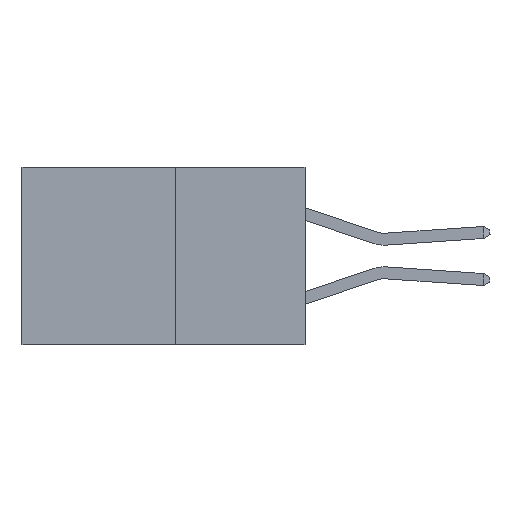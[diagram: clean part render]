
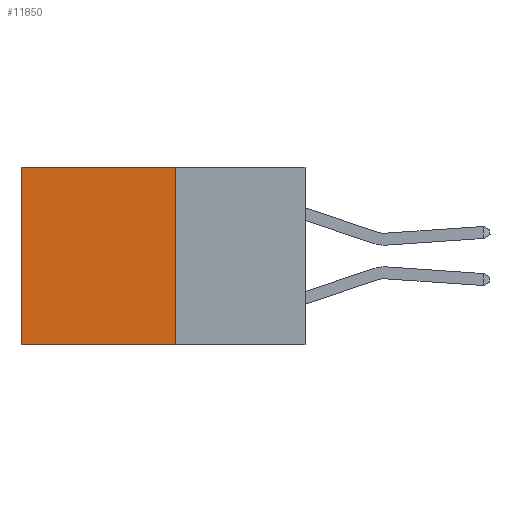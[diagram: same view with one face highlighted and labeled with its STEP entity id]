
A CAD part, left-side view. The second image highlights one B-rep face of the part: STEP entity #11850.
In plain terms, the highlighted planar face has unit normal (-1, 0, 0).
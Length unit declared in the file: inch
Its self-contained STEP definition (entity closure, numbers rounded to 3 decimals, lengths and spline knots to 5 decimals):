
#163 = VECTOR ( 'NONE', #8402, 39.37008 ) ;
#732 = DIRECTION ( 'NONE',  ( 0., 0., -1. ) ) ;
#832 = CARTESIAN_POINT ( 'NONE',  ( 0.277, 0.27, 0. ) ) ;
#913 = CARTESIAN_POINT ( 'NONE',  ( 0.277, 0.27, -0.37 ) ) ;
#1465 = VERTEX_POINT ( 'NONE', #12851 ) ;
#1544 = EDGE_CURVE ( 'NONE', #11478, #1465, #3697, .T. ) ;
#2183 = DIRECTION ( 'NONE',  ( 0., 1., 0. ) ) ;
#2216 = EDGE_CURVE ( 'NONE', #9750, #2980, #11657, .T. ) ;
#2712 = CARTESIAN_POINT ( 'NONE',  ( 0.277, 0.27, 0. ) ) ;
#2980 = VERTEX_POINT ( 'NONE', #5310 ) ;
#3602 = PLANE ( 'NONE',  #3769 ) ;
#3697 = LINE ( 'NONE', #913, #9905 ) ;
#3769 = AXIS2_PLACEMENT_3D ( 'NONE', #8517, #13469, #6119 ) ;
#4355 = ORIENTED_EDGE ( 'NONE', *, *, #1544, .F. ) ;
#5310 = CARTESIAN_POINT ( 'NONE',  ( 0.277, 0.59, 0. ) ) ;
#5454 = VECTOR ( 'NONE', #2183, 39.37008 ) ;
#6108 = ORIENTED_EDGE ( 'NONE', *, *, #2216, .T. ) ;
#6119 = DIRECTION ( 'NONE',  ( 0., 0., -1. ) ) ;
#6754 = CARTESIAN_POINT ( 'NONE',  ( 0.277, 0.27, -0.37 ) ) ;
#6782 = VECTOR ( 'NONE', #732, 39.37008 ) ;
#6860 = LINE ( 'NONE', #14452, #163 ) ;
#7564 = LINE ( 'NONE', #11973, #6782 ) ;
#8402 = DIRECTION ( 'NONE',  ( 0., 0., -1. ) ) ;
#8517 = CARTESIAN_POINT ( 'NONE',  ( 0.277, 0.27, -0.37 ) ) ;
#9184 = FACE_OUTER_BOUND ( 'NONE', #14652, .T. ) ;
#9718 = ORIENTED_EDGE ( 'NONE', *, *, #14774, .T. ) ;
#9750 = VERTEX_POINT ( 'NONE', #832 ) ;
#9905 = VECTOR ( 'NONE', #13828, 39.37008 ) ;
#9961 = ORIENTED_EDGE ( 'NONE', *, *, #10182, .F. ) ;
#10182 = EDGE_CURVE ( 'NONE', #9750, #11478, #6860, .T. ) ;
#11478 = VERTEX_POINT ( 'NONE', #6754 ) ;
#11657 = LINE ( 'NONE', #2712, #5454 ) ;
#11850 = ADVANCED_FACE ( 'NONE', ( #9184 ), #3602, .F. ) ;
#11973 = CARTESIAN_POINT ( 'NONE',  ( 0.277, 0.59, -0.37 ) ) ;
#12851 = CARTESIAN_POINT ( 'NONE',  ( 0.277, 0.59, -0.37 ) ) ;
#13469 = DIRECTION ( 'NONE',  ( 1., 0., 0. ) ) ;
#13828 = DIRECTION ( 'NONE',  ( 0., 1., 0. ) ) ;
#14452 = CARTESIAN_POINT ( 'NONE',  ( 0.277, 0.27, -0.37 ) ) ;
#14652 = EDGE_LOOP ( 'NONE', ( #9718, #4355, #9961, #6108 ) ) ;
#14774 = EDGE_CURVE ( 'NONE', #2980, #1465, #7564, .T. ) ;
